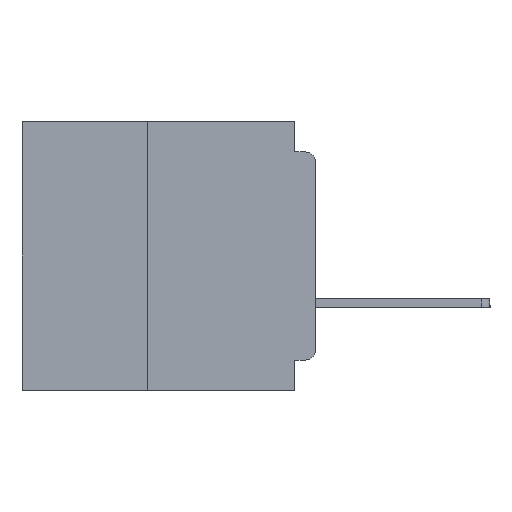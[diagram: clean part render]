
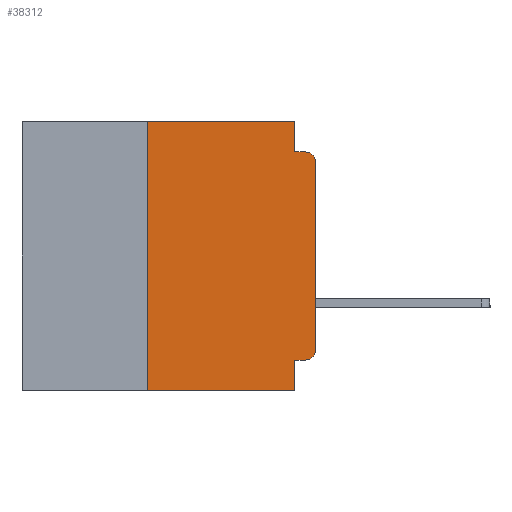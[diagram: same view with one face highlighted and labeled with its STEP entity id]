
A CAD part, left-side view. The second image highlights one B-rep face of the part: STEP entity #38312.
In plain terms, the highlighted planar face has unit normal (-1, 0, 0).
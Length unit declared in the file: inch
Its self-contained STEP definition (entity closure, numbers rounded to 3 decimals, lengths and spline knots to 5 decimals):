
#61 = EDGE_CURVE ( 'NONE', #42804, #29591, #7519, .T. ) ;
#3505 = CARTESIAN_POINT ( 'NONE',  ( 0., 0.015, -0.06 ) ) ;
#4092 = CARTESIAN_POINT ( 'NONE',  ( 0., 0.015, -0.34 ) ) ;
#4273 = VERTEX_POINT ( 'NONE', #23971 ) ;
#4341 = CARTESIAN_POINT ( 'NONE',  ( 0., 0.031, -0.4 ) ) ;
#4522 = VECTOR ( 'NONE', #36936, 39.37008 ) ;
#5061 = CARTESIAN_POINT ( 'NONE',  ( 0., 0.031, 0. ) ) ;
#5192 = EDGE_CURVE ( 'NONE', #40270, #23883, #7683, .T. ) ;
#6197 = LINE ( 'NONE', #52012, #20241 ) ;
#7281 = CARTESIAN_POINT ( 'NONE',  ( 0., 0.031, -0.4 ) ) ;
#7519 = CIRCLE ( 'NONE', #38970, 0.015 ) ;
#7683 = LINE ( 'NONE', #49197, #17705 ) ;
#7856 = DIRECTION ( 'NONE',  ( 0., 0., -1. ) ) ;
#8261 = VECTOR ( 'NONE', #52090, 39.37008 ) ;
#8361 = EDGE_CURVE ( 'NONE', #29591, #48639, #35824, .T. ) ;
#11680 = DIRECTION ( 'NONE',  ( 0., 0., -1. ) ) ;
#12267 = LINE ( 'NONE', #5061, #54687 ) ;
#13522 = AXIS2_PLACEMENT_3D ( 'NONE', #3505, #33283, #7856 ) ;
#14004 = CARTESIAN_POINT ( 'NONE',  ( 0., 0., -0.06 ) ) ;
#14649 = VECTOR ( 'NONE', #19874, 39.37008 ) ;
#14929 = CARTESIAN_POINT ( 'NONE',  ( 0., 0.015, -0.045 ) ) ;
#16982 = ORIENTED_EDGE ( 'NONE', *, *, #51556, .F. ) ;
#17508 = ORIENTED_EDGE ( 'NONE', *, *, #43518, .F. ) ;
#17705 = VECTOR ( 'NONE', #53460, 39.37008 ) ;
#18332 = CIRCLE ( 'NONE', #13522, 0.015 ) ;
#19078 = LINE ( 'NONE', #36059, #52836 ) ;
#19874 = DIRECTION ( 'NONE',  ( 0., 0., 1. ) ) ;
#19976 = EDGE_LOOP ( 'NONE', ( #39331, #22266, #22803, #16982, #40040, #17508, #51738, #24844, #24514, #32009 ) ) ;
#20241 = VECTOR ( 'NONE', #22464, 39.37008 ) ;
#20927 = CARTESIAN_POINT ( 'NONE',  ( 0., 0., -0.355 ) ) ;
#20935 = LINE ( 'NONE', #39291, #8261 ) ;
#22266 = ORIENTED_EDGE ( 'NONE', *, *, #31238, .T. ) ;
#22464 = DIRECTION ( 'NONE',  ( 0., 0., 1. ) ) ;
#22803 = ORIENTED_EDGE ( 'NONE', *, *, #5192, .F. ) ;
#23285 = EDGE_CURVE ( 'NONE', #4273, #36076, #19078, .T. ) ;
#23883 = VERTEX_POINT ( 'NONE', #14929 ) ;
#23971 = CARTESIAN_POINT ( 'NONE',  ( 0., 0.25, -0.4 ) ) ;
#24514 = ORIENTED_EDGE ( 'NONE', *, *, #51959, .F. ) ;
#24720 = CARTESIAN_POINT ( 'NONE',  ( 0., 0.031, -0.045 ) ) ;
#24844 = ORIENTED_EDGE ( 'NONE', *, *, #29096, .F. ) ;
#26536 = DIRECTION ( 'NONE',  ( 0., 0., -1. ) ) ;
#27159 = VERTEX_POINT ( 'NONE', #32271 ) ;
#27533 = CARTESIAN_POINT ( 'NONE',  ( 0., 0., -0.34 ) ) ;
#28597 = PLANE ( 'NONE',  #48021 ) ;
#29096 = EDGE_CURVE ( 'NONE', #27159, #36076, #37076, .T. ) ;
#29591 = VERTEX_POINT ( 'NONE', #27533 ) ;
#31238 = EDGE_CURVE ( 'NONE', #48639, #23883, #18332, .T. ) ;
#32009 = ORIENTED_EDGE ( 'NONE', *, *, #61, .T. ) ;
#32271 = CARTESIAN_POINT ( 'NONE',  ( 0., 0.031, -0.355 ) ) ;
#33283 = DIRECTION ( 'NONE',  ( -1., 0., 0. ) ) ;
#33876 = EDGE_CURVE ( 'NONE', #42394, #50961, #20935, .T. ) ;
#34728 = VECTOR ( 'NONE', #46221, 39.37008 ) ;
#34881 = CARTESIAN_POINT ( 'NONE',  ( 0., 0.25, 0. ) ) ;
#35212 = CARTESIAN_POINT ( 'NONE',  ( 0., 0.031, 0. ) ) ;
#35824 = LINE ( 'NONE', #41110, #14649 ) ;
#36059 = CARTESIAN_POINT ( 'NONE',  ( 0., 0.437, -0.4 ) ) ;
#36076 = VERTEX_POINT ( 'NONE', #4341 ) ;
#36936 = DIRECTION ( 'NONE',  ( 0., 0., -1. ) ) ;
#37022 = DIRECTION ( 'NONE',  ( 1., 0., 0. ) ) ;
#37076 = LINE ( 'NONE', #7281, #4522 ) ;
#37589 = CARTESIAN_POINT ( 'NONE',  ( 0., 0.015, -0.355 ) ) ;
#38312 = ADVANCED_FACE ( 'NONE', ( #41617 ), #28597, .F. ) ;
#38970 = AXIS2_PLACEMENT_3D ( 'NONE', #4092, #42846, #46229 ) ;
#39291 = CARTESIAN_POINT ( 'NONE',  ( 0., 0.437, 0. ) ) ;
#39331 = ORIENTED_EDGE ( 'NONE', *, *, #8361, .T. ) ;
#40040 = ORIENTED_EDGE ( 'NONE', *, *, #33876, .F. ) ;
#40270 = VERTEX_POINT ( 'NONE', #24720 ) ;
#40334 = DIRECTION ( 'NONE',  ( 0., -1., 0. ) ) ;
#41110 = CARTESIAN_POINT ( 'NONE',  ( 0., 0., 0. ) ) ;
#41617 = FACE_OUTER_BOUND ( 'NONE', #19976, .T. ) ;
#42394 = VERTEX_POINT ( 'NONE', #34881 ) ;
#42804 = VERTEX_POINT ( 'NONE', #37589 ) ;
#42846 = DIRECTION ( 'NONE',  ( -1., 0., 0. ) ) ;
#43518 = EDGE_CURVE ( 'NONE', #4273, #42394, #6197, .T. ) ;
#45365 = CARTESIAN_POINT ( 'NONE',  ( 0., 0.437, 0. ) ) ;
#45980 = LINE ( 'NONE', #20927, #34728 ) ;
#46221 = DIRECTION ( 'NONE',  ( 0., 1., 0. ) ) ;
#46229 = DIRECTION ( 'NONE',  ( 0., 0., -1. ) ) ;
#48021 = AXIS2_PLACEMENT_3D ( 'NONE', #45365, #37022, #11680 ) ;
#48639 = VERTEX_POINT ( 'NONE', #14004 ) ;
#49197 = CARTESIAN_POINT ( 'NONE',  ( 0., 0., -0.045 ) ) ;
#50961 = VERTEX_POINT ( 'NONE', #35212 ) ;
#51556 = EDGE_CURVE ( 'NONE', #50961, #40270, #12267, .T. ) ;
#51738 = ORIENTED_EDGE ( 'NONE', *, *, #23285, .T. ) ;
#51959 = EDGE_CURVE ( 'NONE', #42804, #27159, #45980, .T. ) ;
#52012 = CARTESIAN_POINT ( 'NONE',  ( 0., 0.25, -0.4 ) ) ;
#52090 = DIRECTION ( 'NONE',  ( 0., -1., 0. ) ) ;
#52836 = VECTOR ( 'NONE', #40334, 39.37008 ) ;
#53460 = DIRECTION ( 'NONE',  ( 0., -1., 0. ) ) ;
#54687 = VECTOR ( 'NONE', #26536, 39.37008 ) ;
